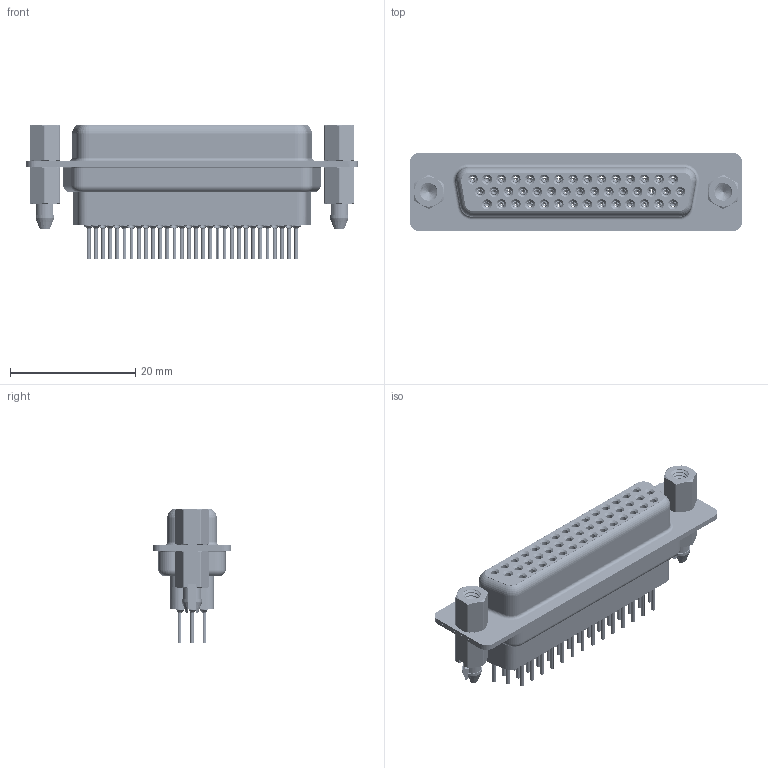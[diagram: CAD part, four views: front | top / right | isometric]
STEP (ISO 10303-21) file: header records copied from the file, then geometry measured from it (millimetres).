
FILE_DESCRIPTION (( 'STEP AP203' ), '1' );
FILE_NAME ('638-044-231-077.STEP', '2020-07-18T22:23:25', ( '' ), ( '' ), 'SwSTEP 2.0', 'SolidWorks 2020', '' );
FILE_SCHEMA (( 'CONFIG_CONTROL_DESIGN' ));
Length unit declared in the file: millimetre
Products named in the file (9): 638 4-40 Threaded Boardlock_LP; 638 Shell Rear_44 Contacts; 638 4-40 Hex Standoff; 638 Contact Row 3_31; 638 Contact Row 1_31; 638-044-231-077; 638 Housing_44 Contacts HP; 638 Shell Front_44 Contacts; 638 Contact Row 2_31
Assembly tree (51 placements, depth 2):
  638-044-231-077
    638 Housing_44 Contacts HP
    638 Shell Front_44 Contacts
    638 Shell Rear_44 Contacts
    638 Contact Row 1_31  x15
    638 Contact Row 2_31  x15
    638 Contact Row 3_31  x14
    638 4-40 Hex Standoff  x2
    638 4-40 Threaded Boardlock_LP  x2
Bounding box: 53.04 x 12.6 x 21.5 mm (x, y, z)
Volume: 4308.5 mm3; surface area: 16120 mm2
Topology: 51 solids, 51 shells, 5891 faces, 15169 edges, 9477 vertices
Faces by surface type: cylinder 1693, plane 1485, torus 1113, bspline 898, cone 702
Entity records: 45584 total; most frequent: CARTESIAN_POINT 14181, DIRECTION 6384, ORIENTED_EDGE 5970, EDGE_CURVE 2985, AXIS2_PLACEMENT_3D 2668, VERTEX_POINT 1895, EDGE_LOOP 1492, CIRCLE 1435
